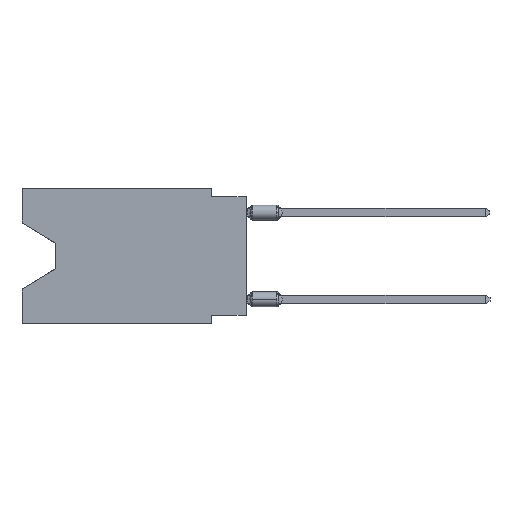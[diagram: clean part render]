
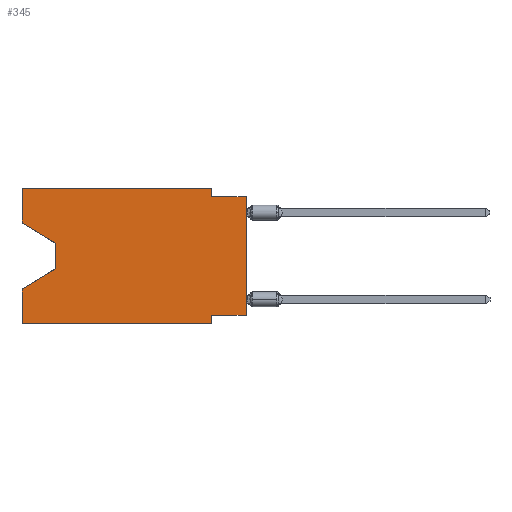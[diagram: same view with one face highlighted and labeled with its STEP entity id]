
A CAD part, left-side view. The second image highlights one B-rep face of the part: STEP entity #345.
In plain terms, the highlighted planar face has unit normal (-1, 0, 0).
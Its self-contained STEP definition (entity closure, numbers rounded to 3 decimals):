
#146 = VERTEX_POINT ( 'NONE', #9643 ) ;
#219 = VECTOR ( 'NONE', #11200, 1000. ) ;
#245 = EDGE_CURVE ( 'NONE', #12250, #15581, #8932, .T. ) ;
#345 = ADVANCED_FACE ( 'NONE', ( #3889 ), #11828, .F. ) ;
#365 = EDGE_CURVE ( 'NONE', #4571, #11442, #9110, .T. ) ;
#698 = EDGE_CURVE ( 'NONE', #4571, #8215, #13888, .T. ) ;
#727 = ORIENTED_EDGE ( 'NONE', *, *, #245, .F. ) ;
#985 = LINE ( 'NONE', #14059, #15900 ) ;
#1030 = EDGE_CURVE ( 'NONE', #7492, #146, #14663, .T. ) ;
#1302 = DIRECTION ( 'NONE',  ( 0., 0., -1. ) ) ;
#1824 = CARTESIAN_POINT ( 'NONE',  ( 0., 13.97, -4.013 ) ) ;
#1987 = ORIENTED_EDGE ( 'NONE', *, *, #4096, .T. ) ;
#2193 = ORIENTED_EDGE ( 'NONE', *, *, #5196, .T. ) ;
#2361 = CARTESIAN_POINT ( 'NONE',  ( 0., 13.97, -5.893 ) ) ;
#2483 = CARTESIAN_POINT ( 'NONE',  ( 0., 16.383, -2.546 ) ) ;
#2502 = CARTESIAN_POINT ( 'NONE',  ( 0., 16.383, 0. ) ) ;
#2590 = VERTEX_POINT ( 'NONE', #5189 ) ;
#2665 = VECTOR ( 'NONE', #12591, 1000. ) ;
#2787 = CARTESIAN_POINT ( 'NONE',  ( 0., 16.383, -7.36 ) ) ;
#3154 = EDGE_CURVE ( 'NONE', #5583, #14851, #9839, .T. ) ;
#3230 = CARTESIAN_POINT ( 'NONE',  ( 0., 0., 0. ) ) ;
#3889 = FACE_OUTER_BOUND ( 'NONE', #16244, .T. ) ;
#4018 = CARTESIAN_POINT ( 'NONE',  ( 0., 13.97, -4.013 ) ) ;
#4056 = VECTOR ( 'NONE', #7790, 1000. ) ;
#4096 = EDGE_CURVE ( 'NONE', #4597, #15581, #12509, .T. ) ;
#4479 = DIRECTION ( 'NONE',  ( 0., -1., 0. ) ) ;
#4571 = VERTEX_POINT ( 'NONE', #14291 ) ;
#4597 = VERTEX_POINT ( 'NONE', #2361 ) ;
#4612 = AXIS2_PLACEMENT_3D ( 'NONE', #9200, #10674, #17095 ) ;
#4744 = EDGE_CURVE ( 'NONE', #2590, #6889, #9566, .T. ) ;
#4752 = CARTESIAN_POINT ( 'NONE',  ( 0., 16.383, -9.906 ) ) ;
#4900 = VECTOR ( 'NONE', #10079, 1000. ) ;
#5023 = ORIENTED_EDGE ( 'NONE', *, *, #698, .F. ) ;
#5167 = ORIENTED_EDGE ( 'NONE', *, *, #14583, .F. ) ;
#5189 = CARTESIAN_POINT ( 'NONE',  ( 0., 2.54, 0. ) ) ;
#5196 = EDGE_CURVE ( 'NONE', #12250, #146, #9697, .T. ) ;
#5583 = VERTEX_POINT ( 'NONE', #9763 ) ;
#5912 = ORIENTED_EDGE ( 'NONE', *, *, #3154, .T. ) ;
#6236 = EDGE_CURVE ( 'NONE', #8215, #2590, #7984, .T. ) ;
#6297 = VECTOR ( 'NONE', #13528, 1000. ) ;
#6540 = LINE ( 'NONE', #4018, #9069 ) ;
#6889 = VERTEX_POINT ( 'NONE', #12823 ) ;
#7250 = CARTESIAN_POINT ( 'NONE',  ( 0., 16.383, -9.906 ) ) ;
#7492 = VERTEX_POINT ( 'NONE', #13388 ) ;
#7790 = DIRECTION ( 'NONE',  ( 0., -0.855, -0.519 ) ) ;
#7984 = LINE ( 'NONE', #2502, #15386 ) ;
#7991 = CARTESIAN_POINT ( 'NONE',  ( 0., 0., -0.635 ) ) ;
#8215 = VERTEX_POINT ( 'NONE', #12765 ) ;
#8312 = VECTOR ( 'NONE', #4479, 1000. ) ;
#8535 = DIRECTION ( 'NONE',  ( 0., 0., 1. ) ) ;
#8932 = LINE ( 'NONE', #16662, #4900 ) ;
#9069 = VECTOR ( 'NONE', #1302, 1000. ) ;
#9110 = LINE ( 'NONE', #2483, #4056 ) ;
#9200 = CARTESIAN_POINT ( 'NONE',  ( 0., 16.383, 0. ) ) ;
#9382 = DIRECTION ( 'NONE',  ( 0., -1., 0. ) ) ;
#9566 = LINE ( 'NONE', #12372, #10811 ) ;
#9596 = ORIENTED_EDGE ( 'NONE', *, *, #6236, .F. ) ;
#9643 = CARTESIAN_POINT ( 'NONE',  ( 0., 2.54, -9.906 ) ) ;
#9697 = LINE ( 'NONE', #7250, #8312 ) ;
#9754 = CARTESIAN_POINT ( 'NONE',  ( 0., 0., -9.271 ) ) ;
#9763 = CARTESIAN_POINT ( 'NONE',  ( 0., 0., -9.271 ) ) ;
#9839 = LINE ( 'NONE', #3230, #11145 ) ;
#10050 = EDGE_CURVE ( 'NONE', #11442, #4597, #6540, .T. ) ;
#10079 = DIRECTION ( 'NONE',  ( 0., 0., 1. ) ) ;
#10674 = DIRECTION ( 'NONE',  ( 1., 0., 0. ) ) ;
#10749 = ORIENTED_EDGE ( 'NONE', *, *, #10050, .T. ) ;
#10811 = VECTOR ( 'NONE', #16329, 1000. ) ;
#11145 = VECTOR ( 'NONE', #8535, 1000. ) ;
#11160 = LINE ( 'NONE', #9754, #14301 ) ;
#11200 = DIRECTION ( 'NONE',  ( 0., 0.855, -0.519 ) ) ;
#11442 = VERTEX_POINT ( 'NONE', #1824 ) ;
#11828 = PLANE ( 'NONE',  #4612 ) ;
#12232 = CARTESIAN_POINT ( 'NONE',  ( 0., 2.54, -9.906 ) ) ;
#12250 = VERTEX_POINT ( 'NONE', #4752 ) ;
#12372 = CARTESIAN_POINT ( 'NONE',  ( 0., 2.54, 0. ) ) ;
#12509 = LINE ( 'NONE', #16727, #219 ) ;
#12591 = DIRECTION ( 'NONE',  ( 0., 0., 1. ) ) ;
#12631 = ORIENTED_EDGE ( 'NONE', *, *, #12662, .F. ) ;
#12662 = EDGE_CURVE ( 'NONE', #6889, #14851, #985, .T. ) ;
#12765 = CARTESIAN_POINT ( 'NONE',  ( 0., 16.383, 0. ) ) ;
#12823 = CARTESIAN_POINT ( 'NONE',  ( 0., 2.54, -0.635 ) ) ;
#12930 = DIRECTION ( 'NONE',  ( 0., -1., 0. ) ) ;
#12998 = ORIENTED_EDGE ( 'NONE', *, *, #365, .T. ) ;
#13388 = CARTESIAN_POINT ( 'NONE',  ( 0., 2.54, -9.271 ) ) ;
#13528 = DIRECTION ( 'NONE',  ( 0., 0., -1. ) ) ;
#13888 = LINE ( 'NONE', #16641, #2665 ) ;
#14059 = CARTESIAN_POINT ( 'NONE',  ( 0., 0., -0.635 ) ) ;
#14291 = CARTESIAN_POINT ( 'NONE',  ( 0., 16.383, -2.546 ) ) ;
#14301 = VECTOR ( 'NONE', #16166, 1000. ) ;
#14583 = EDGE_CURVE ( 'NONE', #5583, #7492, #11160, .T. ) ;
#14663 = LINE ( 'NONE', #12232, #6297 ) ;
#14851 = VERTEX_POINT ( 'NONE', #7991 ) ;
#15386 = VECTOR ( 'NONE', #9382, 1000. ) ;
#15581 = VERTEX_POINT ( 'NONE', #2787 ) ;
#15900 = VECTOR ( 'NONE', #12930, 1000. ) ;
#16060 = ORIENTED_EDGE ( 'NONE', *, *, #1030, .F. ) ;
#16166 = DIRECTION ( 'NONE',  ( 0., 1., 0. ) ) ;
#16244 = EDGE_LOOP ( 'NONE', ( #12998, #10749, #1987, #727, #2193, #16060, #5167, #5912, #12631, #16869, #9596, #5023 ) ) ;
#16329 = DIRECTION ( 'NONE',  ( 0., 0., -1. ) ) ;
#16641 = CARTESIAN_POINT ( 'NONE',  ( 0., 16.383, 0. ) ) ;
#16662 = CARTESIAN_POINT ( 'NONE',  ( 0., 16.383, 0. ) ) ;
#16727 = CARTESIAN_POINT ( 'NONE',  ( 0., 13.97, -5.893 ) ) ;
#16869 = ORIENTED_EDGE ( 'NONE', *, *, #4744, .F. ) ;
#17095 = DIRECTION ( 'NONE',  ( 0., 0., -1. ) ) ;
